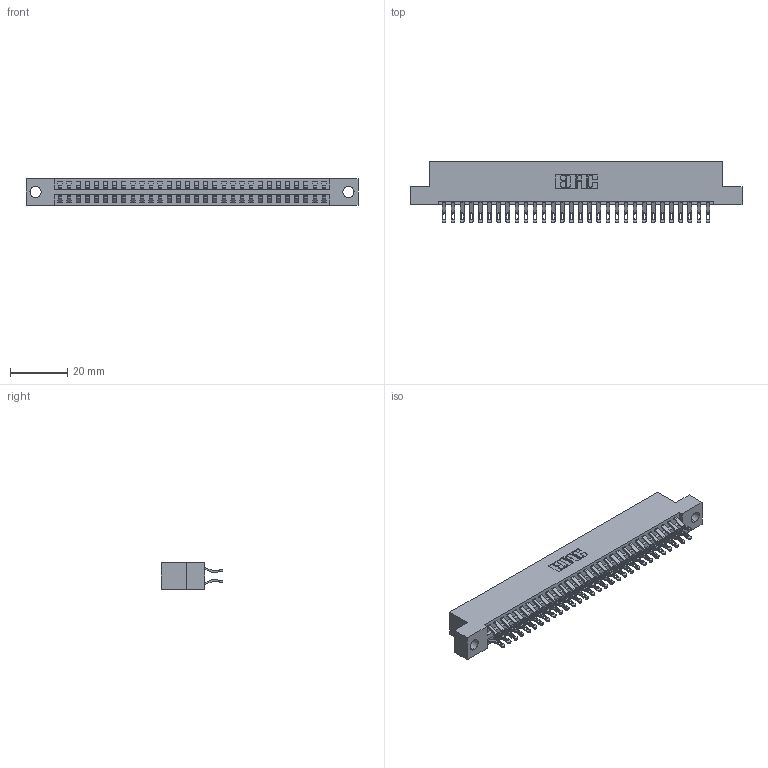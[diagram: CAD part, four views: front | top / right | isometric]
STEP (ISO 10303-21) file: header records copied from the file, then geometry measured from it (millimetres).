
FILE_DESCRIPTION (( 'STEP AP203' ), '1' );
FILE_NAME ('396-060-555-204.STEP', '2018-09-08T13:35:52', ( '' ), ( '' ), 'SwSTEP 2.0', 'SolidWorks 2016', '' );
FILE_SCHEMA (( 'CONFIG_CONTROL_DESIGN' ));
Length unit declared in the file: inch
Products named in the file (3): 346 Part_Flush Mounting Lugs - 0.156 Dia-TH; 345-292-001_555 Tail; 396-060-555-204
Assembly tree (61 placements, depth 2):
  396-060-555-204
    346 Part_Flush Mounting Lugs - 0.156 Dia-TH
    345-292-001_555 Tail  x60
Bounding box: 115.82 x 21.46 x 9.4 mm (x, y, z)
Volume: 11287.3 mm3; surface area: 15760.2 mm2
Topology: 61 solids, 61 shells, 3602 faces, 11309 edges, 7538 vertices
Faces by surface type: plane 2056, cylinder 1546
Entity records: 21523 total; most frequent: CARTESIAN_POINT 3598, ORIENTED_EDGE 3502, DIRECTION 3191, EDGE_CURVE 1751, VECTOR 1479, LINE 1479, VERTEX_POINT 1166, AXIS2_PLACEMENT_3D 856
